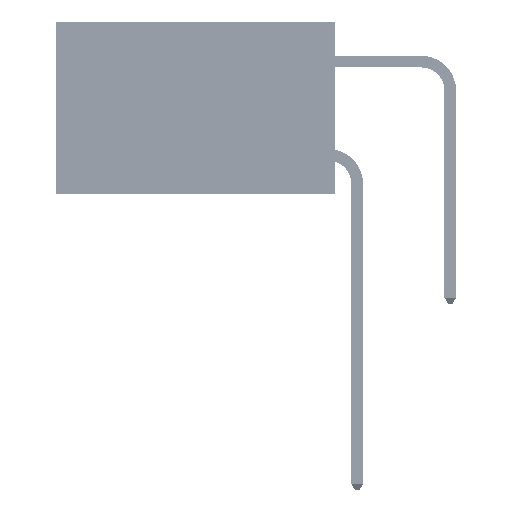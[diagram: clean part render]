
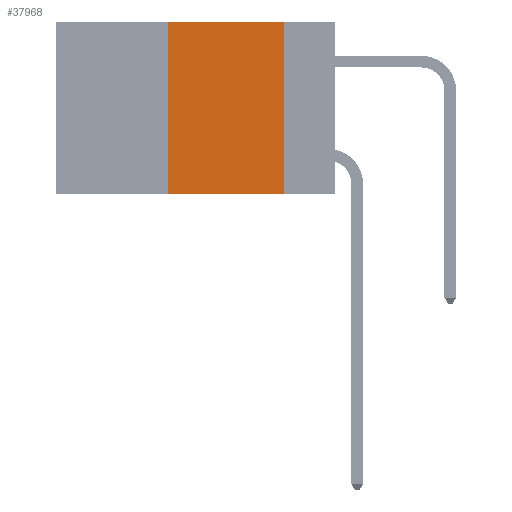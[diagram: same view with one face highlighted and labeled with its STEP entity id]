
A CAD part, left-side view. The second image highlights one B-rep face of the part: STEP entity #37968.
In plain terms, the highlighted planar face has unit normal (-1, 0, 0).
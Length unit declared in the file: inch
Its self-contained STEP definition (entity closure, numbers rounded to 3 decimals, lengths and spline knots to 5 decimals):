
#36 = EDGE_CURVE ( 'NONE', #42439, #33378, #28960, .T. ) ;
#856 = VECTOR ( 'NONE', #21669, 39.37008 ) ;
#3151 = EDGE_LOOP ( 'NONE', ( #37673, #43929, #30248, #36709 ) ) ;
#8955 = VERTEX_POINT ( 'NONE', #9322 ) ;
#9322 = CARTESIAN_POINT ( 'NONE',  ( 0., 0.36, 0. ) ) ;
#11499 = LINE ( 'NONE', #16303, #24785 ) ;
#11763 = VECTOR ( 'NONE', #48004, 39.37008 ) ;
#12418 = VECTOR ( 'NONE', #29750, 39.37008 ) ;
#13862 = DIRECTION ( 'NONE',  ( 1., 0., 0. ) ) ;
#14119 = PLANE ( 'NONE',  #27889 ) ;
#16303 = CARTESIAN_POINT ( 'NONE',  ( 0., 0.6, 0. ) ) ;
#17202 = CARTESIAN_POINT ( 'NONE',  ( 0., 0.36, -0.37 ) ) ;
#20124 = DIRECTION ( 'NONE',  ( 0., -1., 0. ) ) ;
#21669 = DIRECTION ( 'NONE',  ( 0., 0., 1. ) ) ;
#21923 = LINE ( 'NONE', #25736, #856 ) ;
#22436 = VERTEX_POINT ( 'NONE', #17202 ) ;
#23615 = CARTESIAN_POINT ( 'NONE',  ( 0., 0.11, 0. ) ) ;
#24785 = VECTOR ( 'NONE', #20124, 39.37008 ) ;
#25736 = CARTESIAN_POINT ( 'NONE',  ( 0., 0.36, 0. ) ) ;
#27889 = AXIS2_PLACEMENT_3D ( 'NONE', #48657, #13862, #33404 ) ;
#28960 = LINE ( 'NONE', #44442, #11763 ) ;
#29750 = DIRECTION ( 'NONE',  ( 0., -1., 0. ) ) ;
#30248 = ORIENTED_EDGE ( 'NONE', *, *, #32263, .F. ) ;
#32108 = CARTESIAN_POINT ( 'NONE',  ( 0., 0.11, -0.37 ) ) ;
#32263 = EDGE_CURVE ( 'NONE', #22436, #8955, #21923, .T. ) ;
#33378 = VERTEX_POINT ( 'NONE', #32108 ) ;
#33404 = DIRECTION ( 'NONE',  ( 0., 0., -1. ) ) ;
#35322 = EDGE_CURVE ( 'NONE', #22436, #33378, #44485, .T. ) ;
#36709 = ORIENTED_EDGE ( 'NONE', *, *, #35322, .T. ) ;
#37673 = ORIENTED_EDGE ( 'NONE', *, *, #36, .F. ) ;
#37968 = ADVANCED_FACE ( 'NONE', ( #44336 ), #14119, .F. ) ;
#40626 = EDGE_CURVE ( 'NONE', #8955, #42439, #11499, .T. ) ;
#42439 = VERTEX_POINT ( 'NONE', #23615 ) ;
#43929 = ORIENTED_EDGE ( 'NONE', *, *, #40626, .F. ) ;
#44336 = FACE_OUTER_BOUND ( 'NONE', #3151, .T. ) ;
#44442 = CARTESIAN_POINT ( 'NONE',  ( 0., 0.11, 0. ) ) ;
#44485 = LINE ( 'NONE', #44731, #12418 ) ;
#44731 = CARTESIAN_POINT ( 'NONE',  ( 0., 0.6, -0.37 ) ) ;
#48004 = DIRECTION ( 'NONE',  ( 0., 0., -1. ) ) ;
#48657 = CARTESIAN_POINT ( 'NONE',  ( 0., 0.6, 0. ) ) ;
